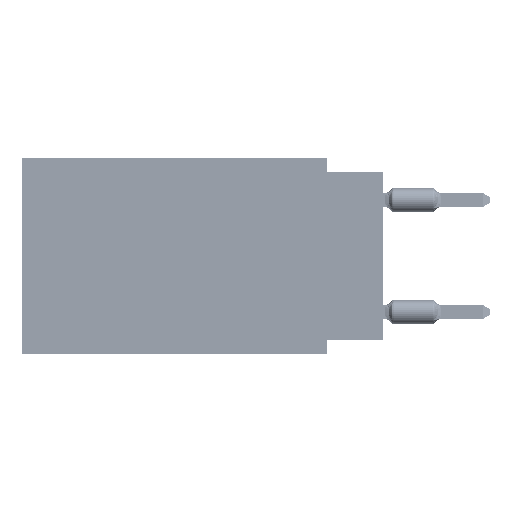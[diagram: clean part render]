
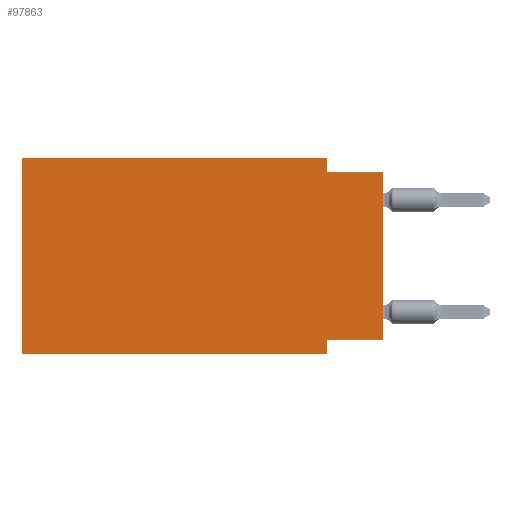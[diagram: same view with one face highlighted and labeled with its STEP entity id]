
A CAD part, left-side view. The second image highlights one B-rep face of the part: STEP entity #97863.
In plain terms, the highlighted planar face has unit normal (-1, 0, 0).
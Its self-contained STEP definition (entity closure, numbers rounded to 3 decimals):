
#799 = EDGE_CURVE ( 'NONE', #66755, #34802, #17150, .T. ) ;
#2524 = CARTESIAN_POINT ( 'NONE',  ( 0., 16.383, 0. ) ) ;
#5409 = EDGE_CURVE ( 'NONE', #53709, #66755, #39241, .T. ) ;
#7366 = CARTESIAN_POINT ( 'NONE',  ( 0., 0., -0.635 ) ) ;
#7381 = DIRECTION ( 'NONE',  ( 0., 1., 0. ) ) ;
#8469 = EDGE_CURVE ( 'NONE', #39753, #33437, #42495, .T. ) ;
#8677 = VERTEX_POINT ( 'NONE', #28820 ) ;
#9711 = CARTESIAN_POINT ( 'NONE',  ( 0., 16.383, -8.89 ) ) ;
#10902 = ORIENTED_EDGE ( 'NONE', *, *, #68825, .F. ) ;
#15255 = VERTEX_POINT ( 'NONE', #82871 ) ;
#15755 = VERTEX_POINT ( 'NONE', #36324 ) ;
#16364 = ORIENTED_EDGE ( 'NONE', *, *, #8469, .F. ) ;
#17150 = LINE ( 'NONE', #7366, #70602 ) ;
#18911 = DIRECTION ( 'NONE',  ( 0., -1., 0. ) ) ;
#20001 = ORIENTED_EDGE ( 'NONE', *, *, #61939, .F. ) ;
#20126 = ORIENTED_EDGE ( 'NONE', *, *, #78771, .T. ) ;
#21172 = LINE ( 'NONE', #36996, #30553 ) ;
#21986 = ORIENTED_EDGE ( 'NONE', *, *, #5409, .F. ) ;
#24083 = ORIENTED_EDGE ( 'NONE', *, *, #45749, .F. ) ;
#24389 = VECTOR ( 'NONE', #7381, 1000. ) ;
#27508 = VECTOR ( 'NONE', #66458, 1000. ) ;
#28820 = CARTESIAN_POINT ( 'NONE',  ( 0., 2.54, -8.89 ) ) ;
#30553 = VECTOR ( 'NONE', #96971, 1000. ) ;
#31423 = AXIS2_PLACEMENT_3D ( 'NONE', #70358, #94919, #52914 ) ;
#33437 = VERTEX_POINT ( 'NONE', #105063 ) ;
#34802 = VERTEX_POINT ( 'NONE', #75054 ) ;
#36324 = CARTESIAN_POINT ( 'NONE',  ( 0., 2.54, -8.255 ) ) ;
#36996 = CARTESIAN_POINT ( 'NONE',  ( 0., 16.383, -8.89 ) ) ;
#39241 = LINE ( 'NONE', #47422, #57139 ) ;
#39753 = VERTEX_POINT ( 'NONE', #9711 ) ;
#40186 = CARTESIAN_POINT ( 'NONE',  ( 0., 2.54, -8.89 ) ) ;
#40525 = VECTOR ( 'NONE', #43038, 1000. ) ;
#40630 = DIRECTION ( 'NONE',  ( 0., -1., 0. ) ) ;
#40665 = VECTOR ( 'NONE', #73453, 1000. ) ;
#40709 = LINE ( 'NONE', #40186, #40665 ) ;
#41366 = CARTESIAN_POINT ( 'NONE',  ( 0., 0., 0. ) ) ;
#42495 = LINE ( 'NONE', #82358, #40525 ) ;
#43038 = DIRECTION ( 'NONE',  ( 0., 0., 1. ) ) ;
#45749 = EDGE_CURVE ( 'NONE', #33437, #53709, #51632, .T. ) ;
#47422 = CARTESIAN_POINT ( 'NONE',  ( 0., 2.54, 0. ) ) ;
#49895 = LINE ( 'NONE', #97946, #24389 ) ;
#50624 = LINE ( 'NONE', #41366, #27508 ) ;
#51632 = LINE ( 'NONE', #2524, #62839 ) ;
#52914 = DIRECTION ( 'NONE',  ( 0., 0., -1. ) ) ;
#53709 = VERTEX_POINT ( 'NONE', #71112 ) ;
#56662 = EDGE_LOOP ( 'NONE', ( #56917, #104487, #21986, #24083, #16364, #20126, #10902, #20001 ) ) ;
#56917 = ORIENTED_EDGE ( 'NONE', *, *, #81865, .T. ) ;
#57139 = VECTOR ( 'NONE', #90516, 1000. ) ;
#61939 = EDGE_CURVE ( 'NONE', #15255, #15755, #49895, .T. ) ;
#62839 = VECTOR ( 'NONE', #18911, 1000. ) ;
#66458 = DIRECTION ( 'NONE',  ( 0., 0., 1. ) ) ;
#66755 = VERTEX_POINT ( 'NONE', #101347 ) ;
#68825 = EDGE_CURVE ( 'NONE', #15755, #8677, #40709, .T. ) ;
#70358 = CARTESIAN_POINT ( 'NONE',  ( 0., 16.383, 0. ) ) ;
#70602 = VECTOR ( 'NONE', #40630, 1000. ) ;
#71112 = CARTESIAN_POINT ( 'NONE',  ( 0., 2.54, 0. ) ) ;
#73453 = DIRECTION ( 'NONE',  ( 0., 0., -1. ) ) ;
#75054 = CARTESIAN_POINT ( 'NONE',  ( 0., 0., -0.635 ) ) ;
#78561 = FACE_OUTER_BOUND ( 'NONE', #56662, .T. ) ;
#78771 = EDGE_CURVE ( 'NONE', #39753, #8677, #21172, .T. ) ;
#81865 = EDGE_CURVE ( 'NONE', #15255, #34802, #50624, .T. ) ;
#82358 = CARTESIAN_POINT ( 'NONE',  ( 0., 16.383, 0. ) ) ;
#82871 = CARTESIAN_POINT ( 'NONE',  ( 0., 0., -8.255 ) ) ;
#90516 = DIRECTION ( 'NONE',  ( 0., 0., -1. ) ) ;
#94919 = DIRECTION ( 'NONE',  ( 1., 0., 0. ) ) ;
#96971 = DIRECTION ( 'NONE',  ( 0., -1., 0. ) ) ;
#97863 = ADVANCED_FACE ( 'NONE', ( #78561 ), #104168, .F. ) ;
#97946 = CARTESIAN_POINT ( 'NONE',  ( 0., 0., -8.255 ) ) ;
#101347 = CARTESIAN_POINT ( 'NONE',  ( 0., 2.54, -0.635 ) ) ;
#104168 = PLANE ( 'NONE',  #31423 ) ;
#104487 = ORIENTED_EDGE ( 'NONE', *, *, #799, .F. ) ;
#105063 = CARTESIAN_POINT ( 'NONE',  ( 0., 16.383, 0. ) ) ;
